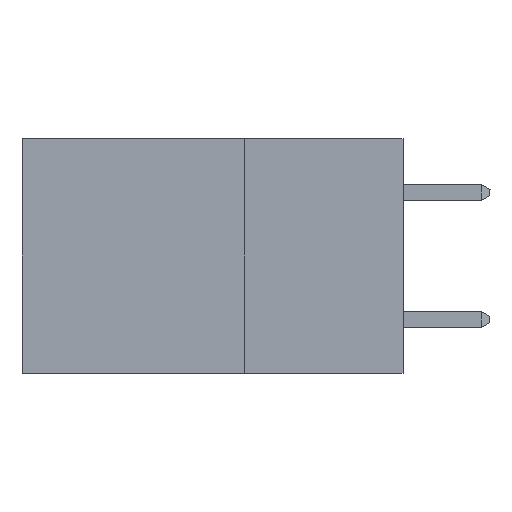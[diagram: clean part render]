
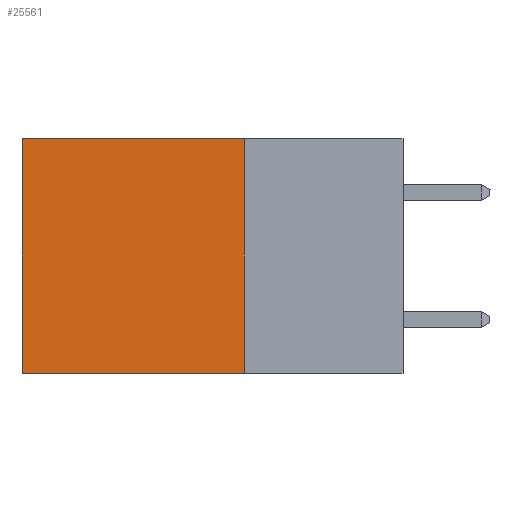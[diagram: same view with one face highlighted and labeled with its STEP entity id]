
A CAD part, left-side view. The second image highlights one B-rep face of the part: STEP entity #25561.
In plain terms, the highlighted planar face has unit normal (-1, 0, 0).
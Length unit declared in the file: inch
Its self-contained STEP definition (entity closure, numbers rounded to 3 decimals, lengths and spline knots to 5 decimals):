
#2754 = VECTOR ( 'NONE', #4827, 39.37008 ) ;
#2804 = EDGE_LOOP ( 'NONE', ( #13902, #10375, #20475, #19311 ) ) ;
#2936 = VECTOR ( 'NONE', #24896, 39.37008 ) ;
#3583 = EDGE_CURVE ( 'NONE', #18307, #6840, #6510, .T. ) ;
#3927 = AXIS2_PLACEMENT_3D ( 'NONE', #20918, #10240, #18587 ) ;
#4827 = DIRECTION ( 'NONE',  ( 0., 1., 0. ) ) ;
#4919 = DIRECTION ( 'NONE',  ( 0., 0., -1. ) ) ;
#6510 = LINE ( 'NONE', #8261, #2936 ) ;
#6840 = VERTEX_POINT ( 'NONE', #26838 ) ;
#7928 = EDGE_CURVE ( 'NONE', #6840, #23995, #23082, .T. ) ;
#8261 = CARTESIAN_POINT ( 'NONE',  ( 0.2875, 0.25, 0. ) ) ;
#8846 = VECTOR ( 'NONE', #4919, 39.37008 ) ;
#9297 = CARTESIAN_POINT ( 'NONE',  ( 0.2875, 0.25, 0. ) ) ;
#10240 = DIRECTION ( 'NONE',  ( 1., 0., 0. ) ) ;
#10375 = ORIENTED_EDGE ( 'NONE', *, *, #7928, .F. ) ;
#11590 = EDGE_CURVE ( 'NONE', #18307, #14704, #19687, .T. ) ;
#13902 = ORIENTED_EDGE ( 'NONE', *, *, #15933, .T. ) ;
#14330 = PLANE ( 'NONE',  #3927 ) ;
#14704 = VERTEX_POINT ( 'NONE', #18223 ) ;
#15933 = EDGE_CURVE ( 'NONE', #14704, #23995, #25656, .T. ) ;
#16522 = DIRECTION ( 'NONE',  ( 0., 1., 0. ) ) ;
#18223 = CARTESIAN_POINT ( 'NONE',  ( 0.2875, 0.6, 0. ) ) ;
#18307 = VERTEX_POINT ( 'NONE', #25877 ) ;
#18587 = DIRECTION ( 'NONE',  ( 0., 0., -1. ) ) ;
#19311 = ORIENTED_EDGE ( 'NONE', *, *, #11590, .T. ) ;
#19687 = LINE ( 'NONE', #9297, #2754 ) ;
#20221 = CARTESIAN_POINT ( 'NONE',  ( 0.2875, 0.6, -0.37 ) ) ;
#20475 = ORIENTED_EDGE ( 'NONE', *, *, #3583, .F. ) ;
#20918 = CARTESIAN_POINT ( 'NONE',  ( 0.2875, 0.25, 0. ) ) ;
#21064 = CARTESIAN_POINT ( 'NONE',  ( 0.2875, 0.25, -0.37 ) ) ;
#23082 = LINE ( 'NONE', #21064, #23381 ) ;
#23381 = VECTOR ( 'NONE', #16522, 39.37008 ) ;
#23995 = VERTEX_POINT ( 'NONE', #20221 ) ;
#24896 = DIRECTION ( 'NONE',  ( 0., 0., -1. ) ) ;
#25561 = ADVANCED_FACE ( 'NONE', ( #26755 ), #14330, .F. ) ;
#25656 = LINE ( 'NONE', #25786, #8846 ) ;
#25786 = CARTESIAN_POINT ( 'NONE',  ( 0.2875, 0.6, 0. ) ) ;
#25877 = CARTESIAN_POINT ( 'NONE',  ( 0.2875, 0.25, 0. ) ) ;
#26755 = FACE_OUTER_BOUND ( 'NONE', #2804, .T. ) ;
#26838 = CARTESIAN_POINT ( 'NONE',  ( 0.2875, 0.25, -0.37 ) ) ;
